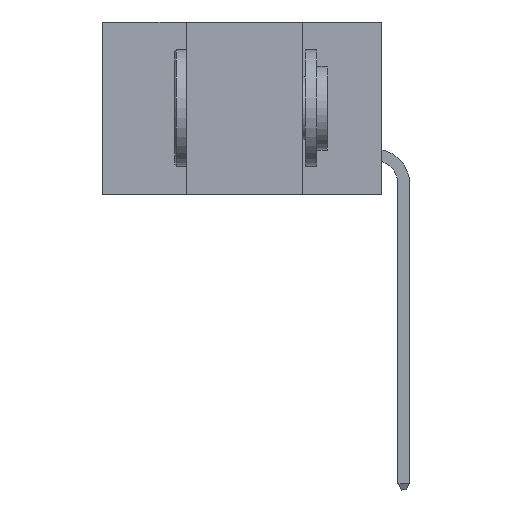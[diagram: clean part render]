
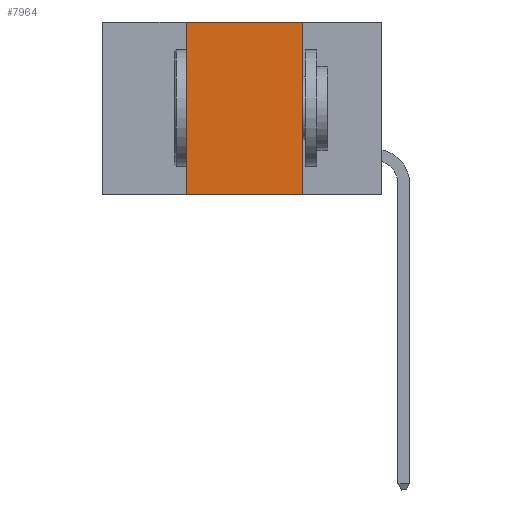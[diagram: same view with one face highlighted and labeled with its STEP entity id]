
A CAD part, left-side view. The second image highlights one B-rep face of the part: STEP entity #7964.
In plain terms, the highlighted planar face has unit normal (-1, 0, 0).
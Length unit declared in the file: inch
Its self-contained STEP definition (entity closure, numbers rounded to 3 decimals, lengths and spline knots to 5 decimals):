
#1997 = FACE_OUTER_BOUND ( 'NONE', #18465, .T. ) ;
#2263 = LINE ( 'NONE', #10186, #14840 ) ;
#2510 = EDGE_CURVE ( 'NONE', #7931, #8973, #22906, .T. ) ;
#3346 = DIRECTION ( 'NONE',  ( 0., 0., -1. ) ) ;
#4788 = DIRECTION ( 'NONE',  ( 0., 0., 1. ) ) ;
#5000 = CARTESIAN_POINT ( 'NONE',  ( 0., 0.17, -0.37 ) ) ;
#5890 = ORIENTED_EDGE ( 'NONE', *, *, #20762, .F. ) ;
#6137 = VERTEX_POINT ( 'NONE', #8344 ) ;
#6649 = VECTOR ( 'NONE', #18473, 39.37008 ) ;
#7872 = EDGE_CURVE ( 'NONE', #6137, #8973, #2263, .T. ) ;
#7931 = VERTEX_POINT ( 'NONE', #13496 ) ;
#7964 = ADVANCED_FACE ( 'NONE', ( #1997 ), #17549, .F. ) ;
#8344 = CARTESIAN_POINT ( 'NONE',  ( 0., 0.42, -0.37 ) ) ;
#8973 = VERTEX_POINT ( 'NONE', #5000 ) ;
#10186 = CARTESIAN_POINT ( 'NONE',  ( 0., 0.6, -0.37 ) ) ;
#10323 = ORIENTED_EDGE ( 'NONE', *, *, #7872, .T. ) ;
#10382 = CARTESIAN_POINT ( 'NONE',  ( 0., 0.6, 0. ) ) ;
#11119 = VECTOR ( 'NONE', #15094, 39.37008 ) ;
#13496 = CARTESIAN_POINT ( 'NONE',  ( 0., 0.17, 0. ) ) ;
#13655 = VECTOR ( 'NONE', #4788, 39.37008 ) ;
#14840 = VECTOR ( 'NONE', #15580, 39.37008 ) ;
#15094 = DIRECTION ( 'NONE',  ( 0., -1., 0. ) ) ;
#15580 = DIRECTION ( 'NONE',  ( 0., -1., 0. ) ) ;
#16888 = CARTESIAN_POINT ( 'NONE',  ( 0., 0.6, 0. ) ) ;
#17549 = PLANE ( 'NONE',  #18337 ) ;
#18337 = AXIS2_PLACEMENT_3D ( 'NONE', #10382, #22922, #3346 ) ;
#18465 = EDGE_LOOP ( 'NONE', ( #21167, #5890, #19525, #10323 ) ) ;
#18473 = DIRECTION ( 'NONE',  ( 0., 0., -1. ) ) ;
#19238 = LINE ( 'NONE', #16888, #11119 ) ;
#19525 = ORIENTED_EDGE ( 'NONE', *, *, #21308, .F. ) ;
#19889 = CARTESIAN_POINT ( 'NONE',  ( 0., 0.17, 0. ) ) ;
#20173 = VERTEX_POINT ( 'NONE', #20509 ) ;
#20509 = CARTESIAN_POINT ( 'NONE',  ( 0., 0.42, 0. ) ) ;
#20762 = EDGE_CURVE ( 'NONE', #20173, #7931, #19238, .T. ) ;
#20809 = CARTESIAN_POINT ( 'NONE',  ( 0., 0.42, 0. ) ) ;
#21167 = ORIENTED_EDGE ( 'NONE', *, *, #2510, .F. ) ;
#21308 = EDGE_CURVE ( 'NONE', #6137, #20173, #22637, .T. ) ;
#22637 = LINE ( 'NONE', #20809, #13655 ) ;
#22906 = LINE ( 'NONE', #19889, #6649 ) ;
#22922 = DIRECTION ( 'NONE',  ( 1., 0., 0. ) ) ;
